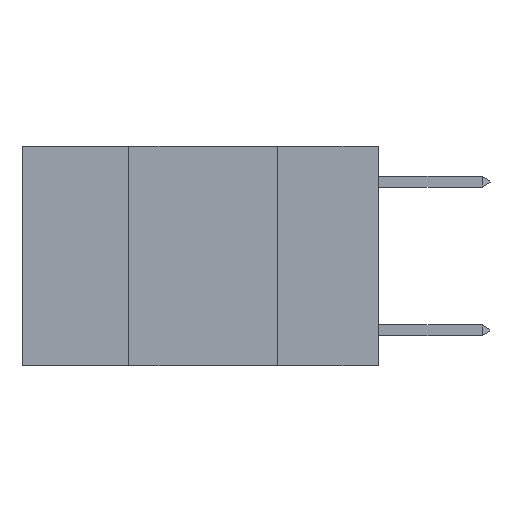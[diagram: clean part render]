
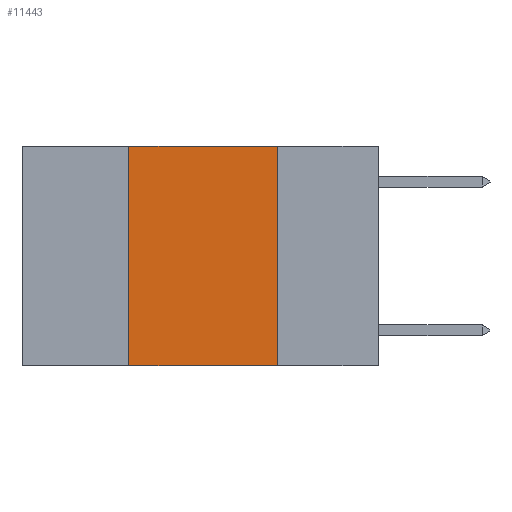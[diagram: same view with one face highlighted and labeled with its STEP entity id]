
A CAD part, left-side view. The second image highlights one B-rep face of the part: STEP entity #11443.
In plain terms, the highlighted planar face has unit normal (-1, 0, 0).
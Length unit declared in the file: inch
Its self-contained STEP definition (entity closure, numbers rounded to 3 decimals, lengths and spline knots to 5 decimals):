
#16 = LINE ( 'NONE', #2973, #6881 ) ;
#116 = VECTOR ( 'NONE', #7763, 39.37008 ) ;
#651 = VERTEX_POINT ( 'NONE', #6130 ) ;
#827 = EDGE_CURVE ( 'NONE', #1268, #651, #5016, .T. ) ;
#1268 = VERTEX_POINT ( 'NONE', #12338 ) ;
#1356 = CARTESIAN_POINT ( 'NONE',  ( 0., 0.6, 0. ) ) ;
#1618 = CARTESIAN_POINT ( 'NONE',  ( 0., 0.17, -0.37 ) ) ;
#2175 = DIRECTION ( 'NONE',  ( 0., 0., 1. ) ) ;
#2399 = PLANE ( 'NONE',  #13195 ) ;
#2973 = CARTESIAN_POINT ( 'NONE',  ( 0., 0.6, -0.37 ) ) ;
#4612 = VERTEX_POINT ( 'NONE', #1618 ) ;
#4793 = VECTOR ( 'NONE', #12142, 39.37008 ) ;
#5016 = LINE ( 'NONE', #13258, #4793 ) ;
#5588 = ORIENTED_EDGE ( 'NONE', *, *, #6240, .F. ) ;
#5641 = DIRECTION ( 'NONE',  ( 1., 0., 0. ) ) ;
#5741 = CARTESIAN_POINT ( 'NONE',  ( 0., 0.42, -0.37 ) ) ;
#6130 = CARTESIAN_POINT ( 'NONE',  ( 0., 0.17, 0. ) ) ;
#6240 = EDGE_CURVE ( 'NONE', #8658, #1268, #12309, .T. ) ;
#6881 = VECTOR ( 'NONE', #7282, 39.37008 ) ;
#7194 = CARTESIAN_POINT ( 'NONE',  ( 0., 0.42, 0. ) ) ;
#7229 = EDGE_CURVE ( 'NONE', #8658, #4612, #16, .T. ) ;
#7282 = DIRECTION ( 'NONE',  ( 0., -1., 0. ) ) ;
#7314 = VECTOR ( 'NONE', #2175, 39.37008 ) ;
#7763 = DIRECTION ( 'NONE',  ( 0., 0., -1. ) ) ;
#7950 = ORIENTED_EDGE ( 'NONE', *, *, #9379, .F. ) ;
#8658 = VERTEX_POINT ( 'NONE', #5741 ) ;
#9379 = EDGE_CURVE ( 'NONE', #651, #4612, #11028, .T. ) ;
#9387 = ORIENTED_EDGE ( 'NONE', *, *, #7229, .T. ) ;
#9797 = EDGE_LOOP ( 'NONE', ( #7950, #12933, #5588, #9387 ) ) ;
#9854 = CARTESIAN_POINT ( 'NONE',  ( 0., 0.17, 0. ) ) ;
#10567 = DIRECTION ( 'NONE',  ( 0., 0., -1. ) ) ;
#11028 = LINE ( 'NONE', #9854, #116 ) ;
#11443 = ADVANCED_FACE ( 'NONE', ( #11720 ), #2399, .F. ) ;
#11720 = FACE_OUTER_BOUND ( 'NONE', #9797, .T. ) ;
#12142 = DIRECTION ( 'NONE',  ( 0., -1., 0. ) ) ;
#12309 = LINE ( 'NONE', #7194, #7314 ) ;
#12338 = CARTESIAN_POINT ( 'NONE',  ( 0., 0.42, 0. ) ) ;
#12933 = ORIENTED_EDGE ( 'NONE', *, *, #827, .F. ) ;
#13195 = AXIS2_PLACEMENT_3D ( 'NONE', #1356, #5641, #10567 ) ;
#13258 = CARTESIAN_POINT ( 'NONE',  ( 0., 0.6, 0. ) ) ;
